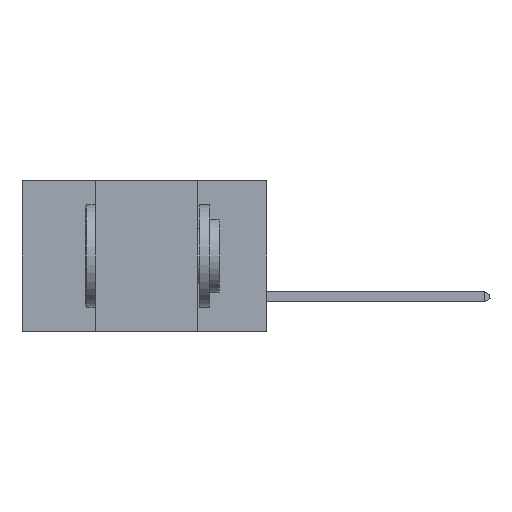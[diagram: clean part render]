
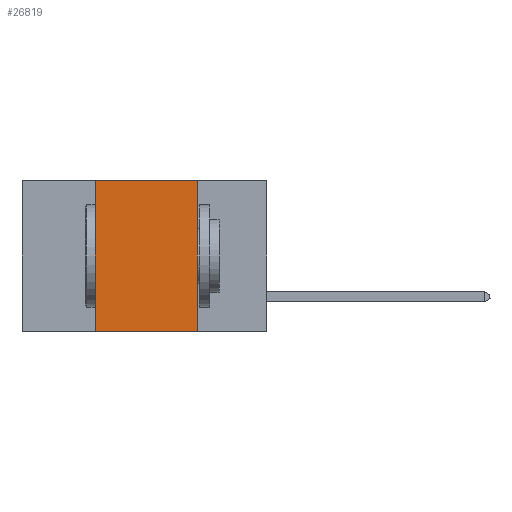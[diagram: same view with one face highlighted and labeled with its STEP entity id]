
A CAD part, left-side view. The second image highlights one B-rep face of the part: STEP entity #26819.
In plain terms, the highlighted planar face has unit normal (-1, 0, 0).
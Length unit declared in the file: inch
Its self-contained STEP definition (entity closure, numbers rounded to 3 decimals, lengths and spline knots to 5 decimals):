
#394 = CARTESIAN_POINT ( 'NONE',  ( 0., 0.6, -0.37 ) ) ;
#701 = CARTESIAN_POINT ( 'NONE',  ( 0., 0.6, 0. ) ) ;
#2128 = AXIS2_PLACEMENT_3D ( 'NONE', #34471, #8826, #34635 ) ;
#3497 = VECTOR ( 'NONE', #46237, 39.37008 ) ;
#4507 = LINE ( 'NONE', #701, #42118 ) ;
#5526 = ORIENTED_EDGE ( 'NONE', *, *, #26522, .F. ) ;
#8491 = FACE_OUTER_BOUND ( 'NONE', #19562, .T. ) ;
#8826 = DIRECTION ( 'NONE',  ( 1., 0., 0. ) ) ;
#9194 = LINE ( 'NONE', #394, #24572 ) ;
#11083 = ORIENTED_EDGE ( 'NONE', *, *, #42508, .F. ) ;
#13414 = LINE ( 'NONE', #25922, #19656 ) ;
#17125 = VERTEX_POINT ( 'NONE', #34599 ) ;
#19562 = EDGE_LOOP ( 'NONE', ( #11083, #5526, #35902, #42022 ) ) ;
#19656 = VECTOR ( 'NONE', #37085, 39.37008 ) ;
#23294 = EDGE_CURVE ( 'NONE', #32210, #36064, #13414, .T. ) ;
#24572 = VECTOR ( 'NONE', #30528, 39.37008 ) ;
#25033 = EDGE_CURVE ( 'NONE', #32210, #44434, #9194, .T. ) ;
#25922 = CARTESIAN_POINT ( 'NONE',  ( 0., 0.42, 0. ) ) ;
#26522 = EDGE_CURVE ( 'NONE', #36064, #17125, #4507, .T. ) ;
#26819 = ADVANCED_FACE ( 'NONE', ( #8491 ), #38289, .F. ) ;
#29635 = CARTESIAN_POINT ( 'NONE',  ( 0., 0.17, -0.37 ) ) ;
#30528 = DIRECTION ( 'NONE',  ( 0., -1., 0. ) ) ;
#31332 = CARTESIAN_POINT ( 'NONE',  ( 0., 0.17, 0. ) ) ;
#32210 = VERTEX_POINT ( 'NONE', #47161 ) ;
#34471 = CARTESIAN_POINT ( 'NONE',  ( 0., 0.6, 0. ) ) ;
#34599 = CARTESIAN_POINT ( 'NONE',  ( 0., 0.17, 0. ) ) ;
#34635 = DIRECTION ( 'NONE',  ( 0., 0., -1. ) ) ;
#35902 = ORIENTED_EDGE ( 'NONE', *, *, #23294, .F. ) ;
#36064 = VERTEX_POINT ( 'NONE', #36151 ) ;
#36151 = CARTESIAN_POINT ( 'NONE',  ( 0., 0.42, 0. ) ) ;
#37085 = DIRECTION ( 'NONE',  ( 0., 0., 1. ) ) ;
#38289 = PLANE ( 'NONE',  #2128 ) ;
#40699 = DIRECTION ( 'NONE',  ( 0., -1., 0. ) ) ;
#42022 = ORIENTED_EDGE ( 'NONE', *, *, #25033, .T. ) ;
#42118 = VECTOR ( 'NONE', #40699, 39.37008 ) ;
#42508 = EDGE_CURVE ( 'NONE', #17125, #44434, #43383, .T. ) ;
#43383 = LINE ( 'NONE', #31332, #3497 ) ;
#44434 = VERTEX_POINT ( 'NONE', #29635 ) ;
#46237 = DIRECTION ( 'NONE',  ( 0., 0., -1. ) ) ;
#47161 = CARTESIAN_POINT ( 'NONE',  ( 0., 0.42, -0.37 ) ) ;
